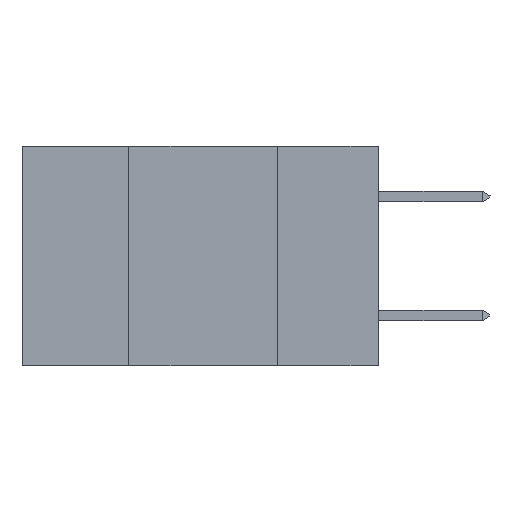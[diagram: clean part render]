
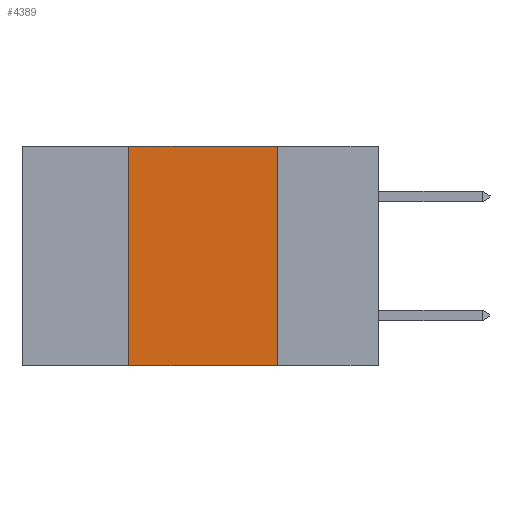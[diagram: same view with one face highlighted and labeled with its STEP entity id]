
A CAD part, left-side view. The second image highlights one B-rep face of the part: STEP entity #4389.
In plain terms, the highlighted planar face has unit normal (-1, 0, 0).
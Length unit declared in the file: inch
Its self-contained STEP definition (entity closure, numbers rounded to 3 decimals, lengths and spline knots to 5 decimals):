
#12 = CARTESIAN_POINT ( 'NONE',  ( 0., 0.17, -0.37 ) ) ;
#29 = LINE ( 'NONE', #5172, #9129 ) ;
#214 = VECTOR ( 'NONE', #1635, 39.37008 ) ;
#741 = ORIENTED_EDGE ( 'NONE', *, *, #1156, .F. ) ;
#1156 = EDGE_CURVE ( 'NONE', #2196, #9795, #9126, .T. ) ;
#1294 = EDGE_CURVE ( 'NONE', #8283, #2196, #29, .T. ) ;
#1339 = EDGE_CURVE ( 'NONE', #7134, #9795, #5062, .T. ) ;
#1635 = DIRECTION ( 'NONE',  ( 0., 0., 1. ) ) ;
#1646 = DIRECTION ( 'NONE',  ( 0., 0., -1. ) ) ;
#1794 = CARTESIAN_POINT ( 'NONE',  ( 0., 0.17, 0. ) ) ;
#1819 = DIRECTION ( 'NONE',  ( 0., -1., 0. ) ) ;
#2123 = EDGE_CURVE ( 'NONE', #7134, #8283, #9220, .T. ) ;
#2196 = VERTEX_POINT ( 'NONE', #1794 ) ;
#2231 = ORIENTED_EDGE ( 'NONE', *, *, #1294, .F. ) ;
#2430 = DIRECTION ( 'NONE',  ( 0., 0., -1. ) ) ;
#2543 = DIRECTION ( 'NONE',  ( 0., -1., 0. ) ) ;
#3346 = CARTESIAN_POINT ( 'NONE',  ( 0., 0.42, -0.37 ) ) ;
#4259 = CARTESIAN_POINT ( 'NONE',  ( 0., 0.42, -0.37 ) ) ;
#4389 = ADVANCED_FACE ( 'NONE', ( #5987 ), #9392, .F. ) ;
#4616 = AXIS2_PLACEMENT_3D ( 'NONE', #8509, #10275, #1646 ) ;
#5062 = LINE ( 'NONE', #8414, #5552 ) ;
#5172 = CARTESIAN_POINT ( 'NONE',  ( 0., 0.6, 0. ) ) ;
#5487 = CARTESIAN_POINT ( 'NONE',  ( 0., 0.42, 0. ) ) ;
#5552 = VECTOR ( 'NONE', #1819, 39.37008 ) ;
#5987 = FACE_OUTER_BOUND ( 'NONE', #6378, .T. ) ;
#6378 = EDGE_LOOP ( 'NONE', ( #741, #2231, #7240, #6817 ) ) ;
#6817 = ORIENTED_EDGE ( 'NONE', *, *, #1339, .T. ) ;
#7134 = VERTEX_POINT ( 'NONE', #4259 ) ;
#7240 = ORIENTED_EDGE ( 'NONE', *, *, #2123, .F. ) ;
#8246 = CARTESIAN_POINT ( 'NONE',  ( 0., 0.17, -0.37 ) ) ;
#8283 = VERTEX_POINT ( 'NONE', #5487 ) ;
#8414 = CARTESIAN_POINT ( 'NONE',  ( 0., 0.6, -0.37 ) ) ;
#8509 = CARTESIAN_POINT ( 'NONE',  ( 0., 0.6, 0. ) ) ;
#9126 = LINE ( 'NONE', #8246, #10383 ) ;
#9129 = VECTOR ( 'NONE', #2543, 39.37008 ) ;
#9220 = LINE ( 'NONE', #3346, #214 ) ;
#9392 = PLANE ( 'NONE',  #4616 ) ;
#9795 = VERTEX_POINT ( 'NONE', #12 ) ;
#10275 = DIRECTION ( 'NONE',  ( 1., 0., 0. ) ) ;
#10383 = VECTOR ( 'NONE', #2430, 39.37008 ) ;
